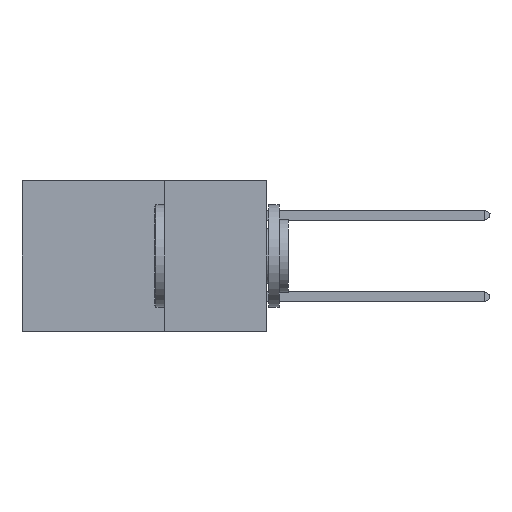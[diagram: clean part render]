
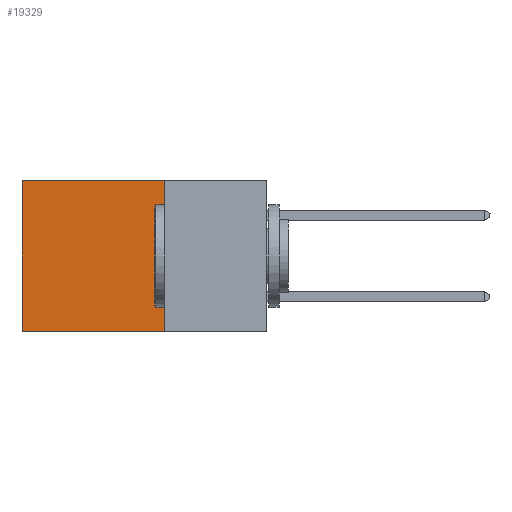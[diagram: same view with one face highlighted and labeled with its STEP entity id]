
A CAD part, left-side view. The second image highlights one B-rep face of the part: STEP entity #19329.
In plain terms, the highlighted planar face has unit normal (-1, 0, 0).
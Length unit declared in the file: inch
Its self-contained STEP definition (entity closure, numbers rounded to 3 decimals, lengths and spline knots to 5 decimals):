
#1984 = VERTEX_POINT ( 'NONE', #4175 ) ;
#2351 = CARTESIAN_POINT ( 'NONE',  ( 0.2875, 0.25, 0. ) ) ;
#2518 = CARTESIAN_POINT ( 'NONE',  ( 0.2875, 0.25, -0.37 ) ) ;
#4175 = CARTESIAN_POINT ( 'NONE',  ( 0.2875, 0.6, 0. ) ) ;
#4231 = VERTEX_POINT ( 'NONE', #27942 ) ;
#4738 = VECTOR ( 'NONE', #12503, 39.37008 ) ;
#5617 = DIRECTION ( 'NONE',  ( 0., 1., 0. ) ) ;
#6959 = EDGE_CURVE ( 'NONE', #4231, #11378, #16062, .T. ) ;
#7168 = VERTEX_POINT ( 'NONE', #2351 ) ;
#8112 = LINE ( 'NONE', #21129, #12262 ) ;
#9767 = AXIS2_PLACEMENT_3D ( 'NONE', #15780, #31749, #18900 ) ;
#11016 = DIRECTION ( 'NONE',  ( 0., 0., -1. ) ) ;
#11378 = VERTEX_POINT ( 'NONE', #17653 ) ;
#11725 = EDGE_CURVE ( 'NONE', #7168, #4231, #16104, .T. ) ;
#12262 = VECTOR ( 'NONE', #5617, 39.37008 ) ;
#12503 = DIRECTION ( 'NONE',  ( 0., 0., -1. ) ) ;
#12534 = EDGE_LOOP ( 'NONE', ( #32365, #20136, #30911, #18576 ) ) ;
#15131 = FACE_OUTER_BOUND ( 'NONE', #12534, .T. ) ;
#15780 = CARTESIAN_POINT ( 'NONE',  ( 0.2875, 0.25, 0. ) ) ;
#16062 = LINE ( 'NONE', #2518, #25186 ) ;
#16104 = LINE ( 'NONE', #21536, #30583 ) ;
#17653 = CARTESIAN_POINT ( 'NONE',  ( 0.2875, 0.6, -0.37 ) ) ;
#18463 = PLANE ( 'NONE',  #9767 ) ;
#18576 = ORIENTED_EDGE ( 'NONE', *, *, #19327, .T. ) ;
#18900 = DIRECTION ( 'NONE',  ( 0., 0., -1. ) ) ;
#19327 = EDGE_CURVE ( 'NONE', #7168, #1984, #8112, .T. ) ;
#19329 = ADVANCED_FACE ( 'NONE', ( #15131 ), #18463, .F. ) ;
#20136 = ORIENTED_EDGE ( 'NONE', *, *, #6959, .F. ) ;
#20571 = DIRECTION ( 'NONE',  ( 0., 1., 0. ) ) ;
#21086 = EDGE_CURVE ( 'NONE', #1984, #11378, #34126, .T. ) ;
#21129 = CARTESIAN_POINT ( 'NONE',  ( 0.2875, 0.25, 0. ) ) ;
#21536 = CARTESIAN_POINT ( 'NONE',  ( 0.2875, 0.25, 0. ) ) ;
#25186 = VECTOR ( 'NONE', #20571, 39.37008 ) ;
#27942 = CARTESIAN_POINT ( 'NONE',  ( 0.2875, 0.25, -0.37 ) ) ;
#30583 = VECTOR ( 'NONE', #11016, 39.37008 ) ;
#30911 = ORIENTED_EDGE ( 'NONE', *, *, #11725, .F. ) ;
#31749 = DIRECTION ( 'NONE',  ( 1., 0., 0. ) ) ;
#32365 = ORIENTED_EDGE ( 'NONE', *, *, #21086, .T. ) ;
#33548 = CARTESIAN_POINT ( 'NONE',  ( 0.2875, 0.6, 0. ) ) ;
#34126 = LINE ( 'NONE', #33548, #4738 ) ;
